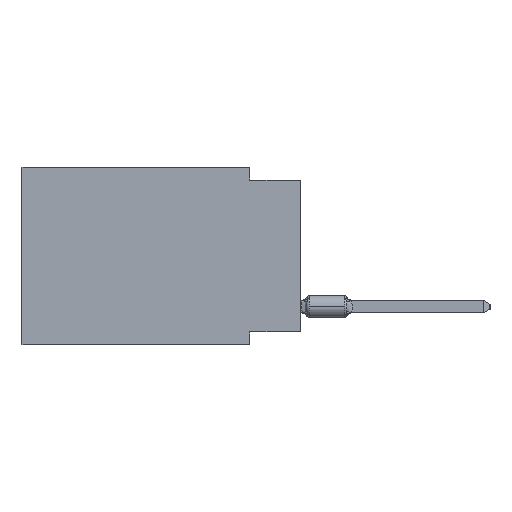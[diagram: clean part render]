
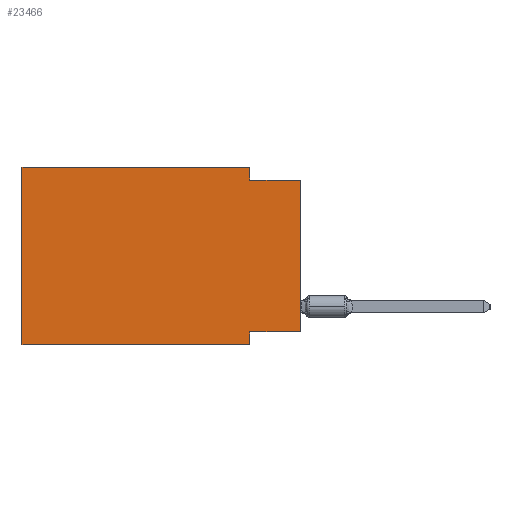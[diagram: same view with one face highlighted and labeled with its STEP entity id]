
A CAD part, left-side view. The second image highlights one B-rep face of the part: STEP entity #23466.
In plain terms, the highlighted planar face has unit normal (-1, 0, 0).
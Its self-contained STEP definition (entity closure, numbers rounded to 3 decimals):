
#1256 = CARTESIAN_POINT ( 'NONE',  ( 0., 13.97, 0. ) ) ;
#1357 = CARTESIAN_POINT ( 'NONE',  ( 0., 2.54, 0. ) ) ;
#1838 = EDGE_CURVE ( 'NONE', #5409, #4379, #17147, .T. ) ;
#2019 = LINE ( 'NONE', #17807, #16698 ) ;
#2124 = ORIENTED_EDGE ( 'NONE', *, *, #26412, .F. ) ;
#2399 = VERTEX_POINT ( 'NONE', #10844 ) ;
#3277 = DIRECTION ( 'NONE',  ( 0., -1., 0. ) ) ;
#3449 = CARTESIAN_POINT ( 'NONE',  ( 0., 2.54, -8.89 ) ) ;
#4379 = VERTEX_POINT ( 'NONE', #1256 ) ;
#4943 = CARTESIAN_POINT ( 'NONE',  ( 0., 13.97, -8.89 ) ) ;
#5018 = VECTOR ( 'NONE', #9775, 1000. ) ;
#5405 = EDGE_CURVE ( 'NONE', #16681, #2399, #23358, .T. ) ;
#5409 = VERTEX_POINT ( 'NONE', #4943 ) ;
#5653 = DIRECTION ( 'NONE',  ( 0., 0., -1. ) ) ;
#7284 = DIRECTION ( 'NONE',  ( 0., 1., 0. ) ) ;
#7525 = LINE ( 'NONE', #20674, #9745 ) ;
#7746 = VERTEX_POINT ( 'NONE', #1357 ) ;
#7972 = CARTESIAN_POINT ( 'NONE',  ( 0., 0., -0.635 ) ) ;
#8406 = PLANE ( 'NONE',  #23811 ) ;
#8534 = CARTESIAN_POINT ( 'NONE',  ( 0., 13.97, 0. ) ) ;
#8708 = LINE ( 'NONE', #28872, #17638 ) ;
#9523 = CARTESIAN_POINT ( 'NONE',  ( 0., 0., -8.255 ) ) ;
#9684 = CARTESIAN_POINT ( 'NONE',  ( 0., 2.54, -8.255 ) ) ;
#9745 = VECTOR ( 'NONE', #3277, 1000. ) ;
#9775 = DIRECTION ( 'NONE',  ( 0., 0., 1. ) ) ;
#10004 = CARTESIAN_POINT ( 'NONE',  ( 0., 2.54, -0.635 ) ) ;
#10357 = ORIENTED_EDGE ( 'NONE', *, *, #5405, .T. ) ;
#10414 = VECTOR ( 'NONE', #5653, 1000. ) ;
#10844 = CARTESIAN_POINT ( 'NONE',  ( 0., 0., -0.635 ) ) ;
#11075 = ORIENTED_EDGE ( 'NONE', *, *, #27536, .F. ) ;
#11274 = VERTEX_POINT ( 'NONE', #9684 ) ;
#11500 = DIRECTION ( 'NONE',  ( 0., 0., -1. ) ) ;
#12373 = LINE ( 'NONE', #7972, #26461 ) ;
#12402 = EDGE_CURVE ( 'NONE', #11274, #25451, #25661, .T. ) ;
#13740 = EDGE_CURVE ( 'NONE', #4379, #7746, #26491, .T. ) ;
#14821 = EDGE_CURVE ( 'NONE', #23682, #2399, #12373, .T. ) ;
#15173 = VECTOR ( 'NONE', #24163, 1000. ) ;
#16035 = ORIENTED_EDGE ( 'NONE', *, *, #12402, .F. ) ;
#16678 = ORIENTED_EDGE ( 'NONE', *, *, #13740, .F. ) ;
#16681 = VERTEX_POINT ( 'NONE', #9523 ) ;
#16698 = VECTOR ( 'NONE', #7284, 1000. ) ;
#16873 = DIRECTION ( 'NONE',  ( 0., -1., 0. ) ) ;
#17147 = LINE ( 'NONE', #8534, #27092 ) ;
#17524 = ORIENTED_EDGE ( 'NONE', *, *, #14821, .F. ) ;
#17638 = VECTOR ( 'NONE', #11500, 1000. ) ;
#17760 = CARTESIAN_POINT ( 'NONE',  ( 0., 13.97, 0. ) ) ;
#17807 = CARTESIAN_POINT ( 'NONE',  ( 0., 0., -8.255 ) ) ;
#18097 = EDGE_LOOP ( 'NONE', ( #10357, #17524, #2124, #16678, #22356, #22268, #16035, #11075 ) ) ;
#18953 = CARTESIAN_POINT ( 'NONE',  ( 0., 0., 0. ) ) ;
#20674 = CARTESIAN_POINT ( 'NONE',  ( 0., 13.97, -8.89 ) ) ;
#21117 = EDGE_CURVE ( 'NONE', #5409, #25451, #7525, .T. ) ;
#21564 = DIRECTION ( 'NONE',  ( 1., 0., 0. ) ) ;
#21643 = CARTESIAN_POINT ( 'NONE',  ( 0., 2.54, -8.89 ) ) ;
#22268 = ORIENTED_EDGE ( 'NONE', *, *, #21117, .T. ) ;
#22356 = ORIENTED_EDGE ( 'NONE', *, *, #1838, .F. ) ;
#23358 = LINE ( 'NONE', #18953, #5018 ) ;
#23466 = ADVANCED_FACE ( 'NONE', ( #24483 ), #8406, .F. ) ;
#23682 = VERTEX_POINT ( 'NONE', #10004 ) ;
#23811 = AXIS2_PLACEMENT_3D ( 'NONE', #17760, #21564, #23904 ) ;
#23904 = DIRECTION ( 'NONE',  ( 0., 0., -1. ) ) ;
#24163 = DIRECTION ( 'NONE',  ( 0., -1., 0. ) ) ;
#24318 = CARTESIAN_POINT ( 'NONE',  ( 0., 13.97, 0. ) ) ;
#24483 = FACE_OUTER_BOUND ( 'NONE', #18097, .T. ) ;
#25451 = VERTEX_POINT ( 'NONE', #21643 ) ;
#25661 = LINE ( 'NONE', #3449, #10414 ) ;
#26412 = EDGE_CURVE ( 'NONE', #7746, #23682, #8708, .T. ) ;
#26461 = VECTOR ( 'NONE', #16873, 1000. ) ;
#26491 = LINE ( 'NONE', #24318, #15173 ) ;
#27092 = VECTOR ( 'NONE', #28250, 1000. ) ;
#27536 = EDGE_CURVE ( 'NONE', #16681, #11274, #2019, .T. ) ;
#28250 = DIRECTION ( 'NONE',  ( 0., 0., 1. ) ) ;
#28872 = CARTESIAN_POINT ( 'NONE',  ( 0., 2.54, 0. ) ) ;
